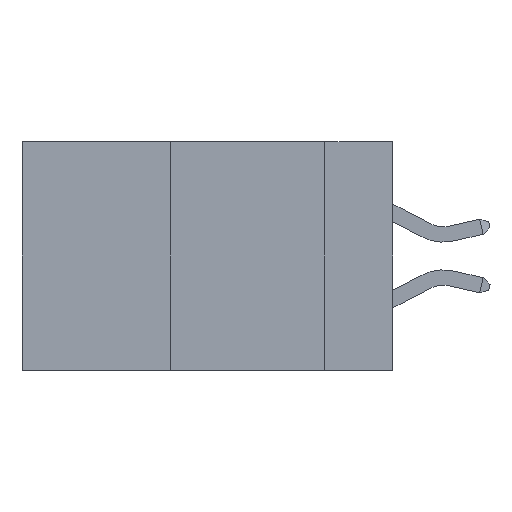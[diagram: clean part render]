
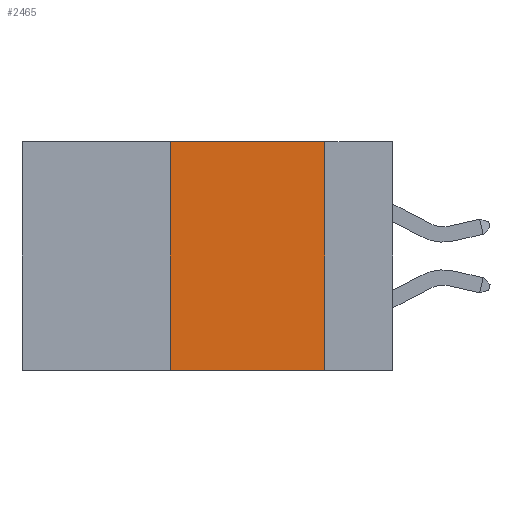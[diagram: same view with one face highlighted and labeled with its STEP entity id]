
A CAD part, left-side view. The second image highlights one B-rep face of the part: STEP entity #2465.
In plain terms, the highlighted planar face has unit normal (-1, 0, 0).
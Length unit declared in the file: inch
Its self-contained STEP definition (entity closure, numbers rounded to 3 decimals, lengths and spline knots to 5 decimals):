
#402 = VECTOR ( 'NONE', #6579, 39.37008 ) ;
#840 = EDGE_CURVE ( 'NONE', #22083, #10961, #12963, .T. ) ;
#1005 = EDGE_CURVE ( 'NONE', #10961, #10871, #1552, .T. ) ;
#1552 = LINE ( 'NONE', #13311, #9710 ) ;
#2421 = DIRECTION ( 'NONE',  ( 0., -1., 0. ) ) ;
#2465 = ADVANCED_FACE ( 'NONE', ( #16104 ), #17051, .F. ) ;
#3966 = CARTESIAN_POINT ( 'NONE',  ( 0., 0.11, -0.37 ) ) ;
#4314 = EDGE_CURVE ( 'NONE', #10871, #13514, #18347, .T. ) ;
#4505 = EDGE_LOOP ( 'NONE', ( #21259, #8788, #9896, #10435 ) ) ;
#4834 = CARTESIAN_POINT ( 'NONE',  ( 0., 0.6, -0.37 ) ) ;
#5949 = CARTESIAN_POINT ( 'NONE',  ( 0., 0.36, 0. ) ) ;
#6579 = DIRECTION ( 'NONE',  ( 0., -1., 0. ) ) ;
#6747 = DIRECTION ( 'NONE',  ( 0., 0., -1. ) ) ;
#8098 = CARTESIAN_POINT ( 'NONE',  ( 0., 0.36, -0.37 ) ) ;
#8461 = DIRECTION ( 'NONE',  ( 0., 0., -1. ) ) ;
#8788 = ORIENTED_EDGE ( 'NONE', *, *, #1005, .F. ) ;
#8980 = DIRECTION ( 'NONE',  ( 0., 0., 1. ) ) ;
#9710 = VECTOR ( 'NONE', #2421, 39.37008 ) ;
#9896 = ORIENTED_EDGE ( 'NONE', *, *, #840, .F. ) ;
#10435 = ORIENTED_EDGE ( 'NONE', *, *, #20348, .T. ) ;
#10871 = VERTEX_POINT ( 'NONE', #14188 ) ;
#10961 = VERTEX_POINT ( 'NONE', #16110 ) ;
#12963 = LINE ( 'NONE', #5949, #16963 ) ;
#13311 = CARTESIAN_POINT ( 'NONE',  ( 0., 0.6, 0. ) ) ;
#13514 = VERTEX_POINT ( 'NONE', #3966 ) ;
#14188 = CARTESIAN_POINT ( 'NONE',  ( 0., 0.11, 0. ) ) ;
#14255 = LINE ( 'NONE', #4834, #402 ) ;
#15396 = CARTESIAN_POINT ( 'NONE',  ( 0., 0.11, 0. ) ) ;
#16104 = FACE_OUTER_BOUND ( 'NONE', #4505, .T. ) ;
#16110 = CARTESIAN_POINT ( 'NONE',  ( 0., 0.36, 0. ) ) ;
#16963 = VECTOR ( 'NONE', #8980, 39.37008 ) ;
#17051 = PLANE ( 'NONE',  #19782 ) ;
#17829 = VECTOR ( 'NONE', #6747, 39.37008 ) ;
#18347 = LINE ( 'NONE', #15396, #17829 ) ;
#18703 = DIRECTION ( 'NONE',  ( 1., 0., 0. ) ) ;
#19782 = AXIS2_PLACEMENT_3D ( 'NONE', #20295, #18703, #8461 ) ;
#20295 = CARTESIAN_POINT ( 'NONE',  ( 0., 0.6, 0. ) ) ;
#20348 = EDGE_CURVE ( 'NONE', #22083, #13514, #14255, .T. ) ;
#21259 = ORIENTED_EDGE ( 'NONE', *, *, #4314, .F. ) ;
#22083 = VERTEX_POINT ( 'NONE', #8098 ) ;
